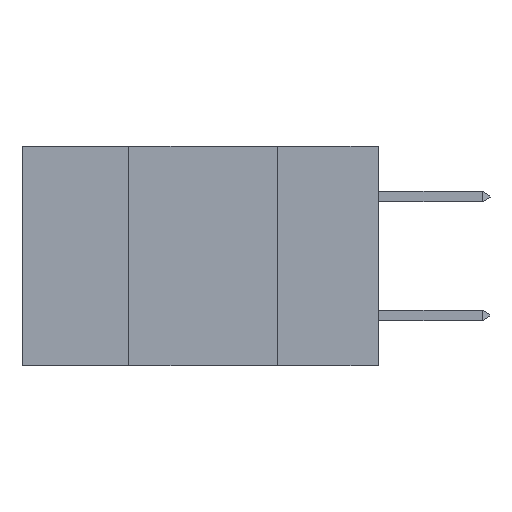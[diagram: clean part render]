
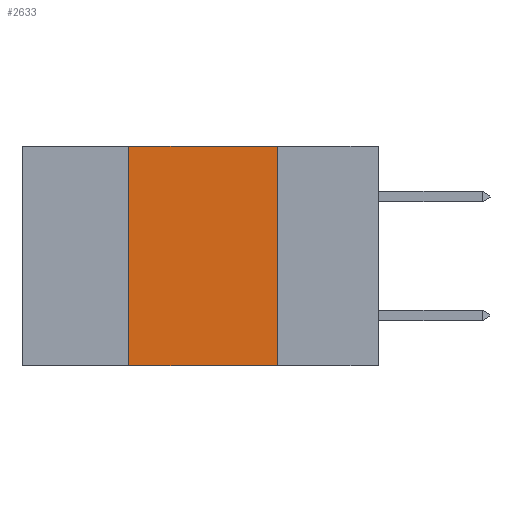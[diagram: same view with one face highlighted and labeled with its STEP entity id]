
A CAD part, left-side view. The second image highlights one B-rep face of the part: STEP entity #2633.
In plain terms, the highlighted planar face has unit normal (-1, 0, 0).
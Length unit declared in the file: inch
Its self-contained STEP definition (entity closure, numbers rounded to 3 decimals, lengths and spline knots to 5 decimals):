
#742 = CARTESIAN_POINT ( 'NONE',  ( 0., 0.42, -0.37 ) ) ;
#1234 = CARTESIAN_POINT ( 'NONE',  ( 0., 0.42, 0. ) ) ;
#1386 = FACE_OUTER_BOUND ( 'NONE', #14020, .T. ) ;
#1587 = ORIENTED_EDGE ( 'NONE', *, *, #9895, .T. ) ;
#2633 = ADVANCED_FACE ( 'NONE', ( #1386 ), #11707, .F. ) ;
#2663 = DIRECTION ( 'NONE',  ( 0., 0., -1. ) ) ;
#3504 = CARTESIAN_POINT ( 'NONE',  ( 0., 0.6, -0.37 ) ) ;
#4891 = CARTESIAN_POINT ( 'NONE',  ( 0., 0.17, 0. ) ) ;
#4971 = VECTOR ( 'NONE', #7646, 39.37008 ) ;
#5028 = EDGE_CURVE ( 'NONE', #15005, #11127, #11394, .T. ) ;
#5840 = LINE ( 'NONE', #16666, #8674 ) ;
#5993 = ORIENTED_EDGE ( 'NONE', *, *, #5028, .F. ) ;
#6189 = ORIENTED_EDGE ( 'NONE', *, *, #14846, .F. ) ;
#7012 = ORIENTED_EDGE ( 'NONE', *, *, #12220, .F. ) ;
#7478 = DIRECTION ( 'NONE',  ( 0., -1., 0. ) ) ;
#7646 = DIRECTION ( 'NONE',  ( 0., -1., 0. ) ) ;
#7801 = VERTEX_POINT ( 'NONE', #4891 ) ;
#8674 = VECTOR ( 'NONE', #2663, 39.37008 ) ;
#9121 = CARTESIAN_POINT ( 'NONE',  ( 0., 0.42, 0. ) ) ;
#9191 = CARTESIAN_POINT ( 'NONE',  ( 0., 0.6, 0. ) ) ;
#9209 = AXIS2_PLACEMENT_3D ( 'NONE', #9191, #15776, #13127 ) ;
#9895 = EDGE_CURVE ( 'NONE', #15005, #11861, #16642, .T. ) ;
#11127 = VERTEX_POINT ( 'NONE', #1234 ) ;
#11394 = LINE ( 'NONE', #9121, #16054 ) ;
#11707 = PLANE ( 'NONE',  #9209 ) ;
#11861 = VERTEX_POINT ( 'NONE', #15703 ) ;
#12220 = EDGE_CURVE ( 'NONE', #7801, #11861, #5840, .T. ) ;
#12235 = LINE ( 'NONE', #15213, #4971 ) ;
#12647 = VECTOR ( 'NONE', #7478, 39.37008 ) ;
#13127 = DIRECTION ( 'NONE',  ( 0., 0., -1. ) ) ;
#13367 = DIRECTION ( 'NONE',  ( 0., 0., 1. ) ) ;
#14020 = EDGE_LOOP ( 'NONE', ( #7012, #6189, #5993, #1587 ) ) ;
#14846 = EDGE_CURVE ( 'NONE', #11127, #7801, #12235, .T. ) ;
#15005 = VERTEX_POINT ( 'NONE', #742 ) ;
#15213 = CARTESIAN_POINT ( 'NONE',  ( 0., 0.6, 0. ) ) ;
#15703 = CARTESIAN_POINT ( 'NONE',  ( 0., 0.17, -0.37 ) ) ;
#15776 = DIRECTION ( 'NONE',  ( 1., 0., 0. ) ) ;
#16054 = VECTOR ( 'NONE', #13367, 39.37008 ) ;
#16642 = LINE ( 'NONE', #3504, #12647 ) ;
#16666 = CARTESIAN_POINT ( 'NONE',  ( 0., 0.17, 0. ) ) ;
